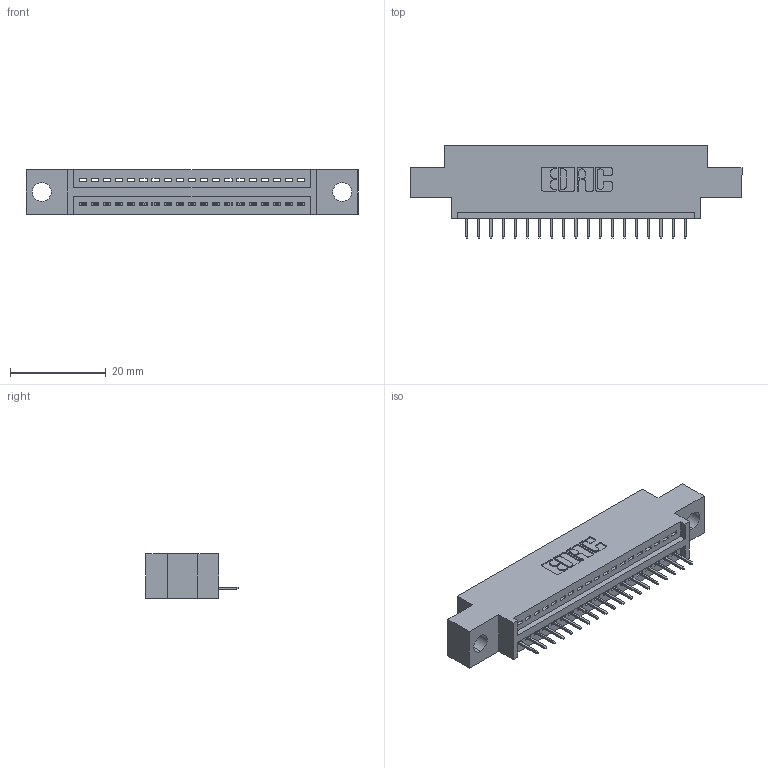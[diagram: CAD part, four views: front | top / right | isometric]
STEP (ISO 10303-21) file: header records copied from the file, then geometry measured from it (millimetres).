
FILE_DESCRIPTION (( 'STEP AP203' ), '1' );
FILE_NAME ('395-019-524-604.STEP', '2021-05-31T14:27:22', ( '' ), ( '' ), 'SwSTEP 2.0', 'SolidWorks 2020', '' );
FILE_SCHEMA (( 'CONFIG_CONTROL_DESIGN' ));
Length unit declared in the file: inch
Products named in the file (3): 395-019-524-604; 345-292-001_345-293-124; 345 Part_0.170 Offset - 0.156 Dia-TI
Assembly tree (20 placements, depth 2):
  395-019-524-604
    345 Part_0.170 Offset - 0.156 Dia-TI
    345-292-001_345-293-124  x19
Bounding box: 69.47 x 19.35 x 9.4 mm (x, y, z)
Volume: 6115.4 mm3; surface area: 7543.3 mm2
Topology: 20 solids, 20 shells, 1322 faces, 3809 edges, 2462 vertices
Faces by surface type: plane 972, cylinder 350
Entity records: 18021 total; most frequent: CARTESIAN_POINT 3131, ORIENTED_EDGE 3082, DIRECTION 2767, EDGE_CURVE 1541, LINE 1337, VECTOR 1337, VERTEX_POINT 1022, AXIS2_PLACEMENT_3D 715
